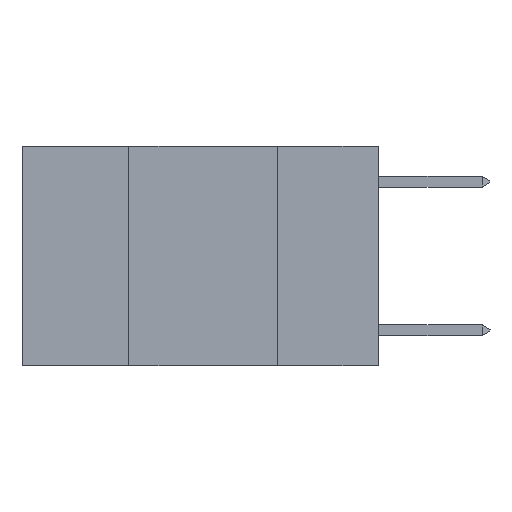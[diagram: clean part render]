
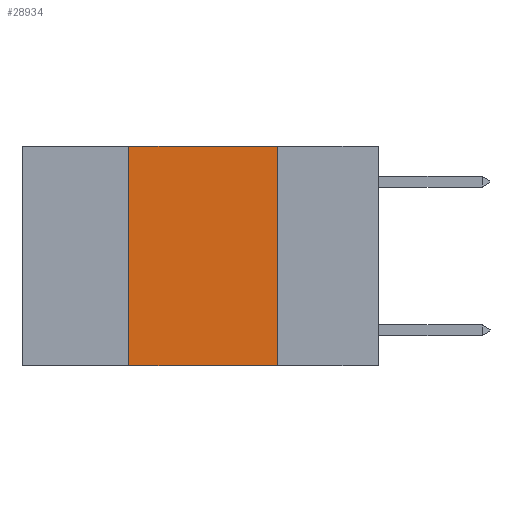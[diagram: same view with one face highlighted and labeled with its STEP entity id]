
A CAD part, left-side view. The second image highlights one B-rep face of the part: STEP entity #28934.
In plain terms, the highlighted planar face has unit normal (-1, 0, 0).
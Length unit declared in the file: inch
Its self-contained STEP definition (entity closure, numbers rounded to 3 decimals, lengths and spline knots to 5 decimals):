
#2306 = FACE_OUTER_BOUND ( 'NONE', #25729, .T. ) ;
#2911 = CARTESIAN_POINT ( 'NONE',  ( 0., 0.6, -0.37 ) ) ;
#3107 = LINE ( 'NONE', #17633, #27171 ) ;
#4253 = VERTEX_POINT ( 'NONE', #4805 ) ;
#4805 = CARTESIAN_POINT ( 'NONE',  ( 0., 0.17, 0. ) ) ;
#6527 = DIRECTION ( 'NONE',  ( 1., 0., 0. ) ) ;
#6907 = DIRECTION ( 'NONE',  ( 0., 0., 1. ) ) ;
#8282 = VECTOR ( 'NONE', #6907, 39.37008 ) ;
#9185 = VECTOR ( 'NONE', #24558, 39.37008 ) ;
#10975 = VERTEX_POINT ( 'NONE', #19582 ) ;
#11700 = CARTESIAN_POINT ( 'NONE',  ( 0., 0.42, 0. ) ) ;
#12163 = AXIS2_PLACEMENT_3D ( 'NONE', #27976, #6527, #23423 ) ;
#14915 = LINE ( 'NONE', #2911, #9185 ) ;
#15813 = CARTESIAN_POINT ( 'NONE',  ( 0., 0.17, -0.37 ) ) ;
#16000 = VECTOR ( 'NONE', #19112, 39.37008 ) ;
#17633 = CARTESIAN_POINT ( 'NONE',  ( 0., 0.6, 0. ) ) ;
#18164 = EDGE_CURVE ( 'NONE', #4253, #30766, #29171, .T. ) ;
#19112 = DIRECTION ( 'NONE',  ( 0., 0., -1. ) ) ;
#19265 = ORIENTED_EDGE ( 'NONE', *, *, #18164, .F. ) ;
#19575 = VERTEX_POINT ( 'NONE', #27774 ) ;
#19582 = CARTESIAN_POINT ( 'NONE',  ( 0., 0.42, 0. ) ) ;
#21099 = PLANE ( 'NONE',  #12163 ) ;
#21185 = ORIENTED_EDGE ( 'NONE', *, *, #29949, .F. ) ;
#21502 = ORIENTED_EDGE ( 'NONE', *, *, #25213, .F. ) ;
#23423 = DIRECTION ( 'NONE',  ( 0., 0., -1. ) ) ;
#24558 = DIRECTION ( 'NONE',  ( 0., -1., 0. ) ) ;
#25213 = EDGE_CURVE ( 'NONE', #19575, #10975, #27365, .T. ) ;
#25729 = EDGE_LOOP ( 'NONE', ( #19265, #21185, #21502, #29460 ) ) ;
#27171 = VECTOR ( 'NONE', #29350, 39.37008 ) ;
#27365 = LINE ( 'NONE', #11700, #8282 ) ;
#27774 = CARTESIAN_POINT ( 'NONE',  ( 0., 0.42, -0.37 ) ) ;
#27976 = CARTESIAN_POINT ( 'NONE',  ( 0., 0.6, 0. ) ) ;
#28934 = ADVANCED_FACE ( 'NONE', ( #2306 ), #21099, .F. ) ;
#29171 = LINE ( 'NONE', #30578, #16000 ) ;
#29350 = DIRECTION ( 'NONE',  ( 0., -1., 0. ) ) ;
#29460 = ORIENTED_EDGE ( 'NONE', *, *, #30589, .T. ) ;
#29949 = EDGE_CURVE ( 'NONE', #10975, #4253, #3107, .T. ) ;
#30578 = CARTESIAN_POINT ( 'NONE',  ( 0., 0.17, 0. ) ) ;
#30589 = EDGE_CURVE ( 'NONE', #19575, #30766, #14915, .T. ) ;
#30766 = VERTEX_POINT ( 'NONE', #15813 ) ;
